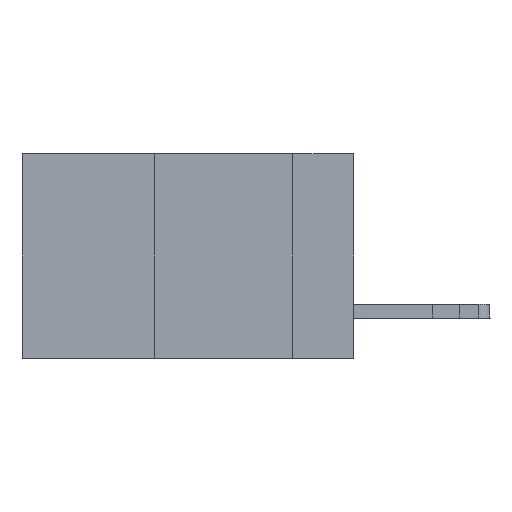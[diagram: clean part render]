
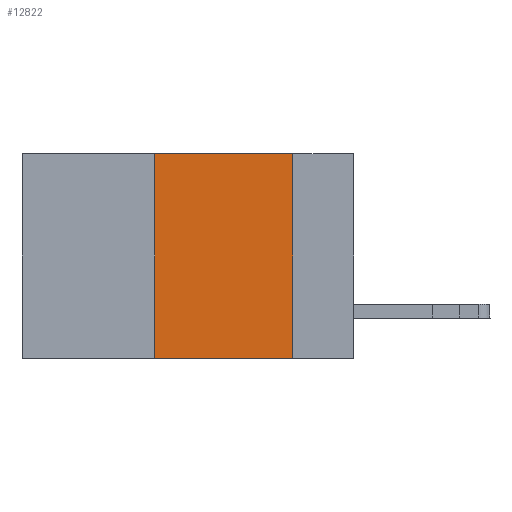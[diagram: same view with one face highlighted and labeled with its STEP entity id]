
A CAD part, left-side view. The second image highlights one B-rep face of the part: STEP entity #12822.
In plain terms, the highlighted planar face has unit normal (-1, 0, 0).
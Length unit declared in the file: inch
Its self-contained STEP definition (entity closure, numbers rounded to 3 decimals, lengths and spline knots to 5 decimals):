
#306 = ORIENTED_EDGE ( 'NONE', *, *, #20169, .F. ) ;
#942 = FACE_OUTER_BOUND ( 'NONE', #16333, .T. ) ;
#2393 = VERTEX_POINT ( 'NONE', #7620 ) ;
#2724 = PLANE ( 'NONE',  #6733 ) ;
#3853 = LINE ( 'NONE', #5769, #23176 ) ;
#4171 = ORIENTED_EDGE ( 'NONE', *, *, #15342, .F. ) ;
#5148 = VECTOR ( 'NONE', #10965, 39.37008 ) ;
#5769 = CARTESIAN_POINT ( 'NONE',  ( 0., 0.36, 0. ) ) ;
#5931 = VERTEX_POINT ( 'NONE', #22778 ) ;
#6733 = AXIS2_PLACEMENT_3D ( 'NONE', #22845, #21169, #19491 ) ;
#7384 = LINE ( 'NONE', #9068, #5148 ) ;
#7620 = CARTESIAN_POINT ( 'NONE',  ( 0., 0.36, 0. ) ) ;
#7730 = CARTESIAN_POINT ( 'NONE',  ( 0., 0.11, 0. ) ) ;
#7844 = VERTEX_POINT ( 'NONE', #20272 ) ;
#8581 = CARTESIAN_POINT ( 'NONE',  ( 0., 0.11, -0.37 ) ) ;
#8760 = ORIENTED_EDGE ( 'NONE', *, *, #23398, .F. ) ;
#9068 = CARTESIAN_POINT ( 'NONE',  ( 0., 0.6, -0.37 ) ) ;
#9505 = VECTOR ( 'NONE', #17516, 39.37008 ) ;
#10965 = DIRECTION ( 'NONE',  ( 0., -1., 0. ) ) ;
#11073 = VERTEX_POINT ( 'NONE', #8581 ) ;
#11653 = DIRECTION ( 'NONE',  ( 0., 0., -1. ) ) ;
#11854 = ORIENTED_EDGE ( 'NONE', *, *, #14132, .T. ) ;
#12822 = ADVANCED_FACE ( 'NONE', ( #942 ), #2724, .F. ) ;
#13293 = DIRECTION ( 'NONE',  ( 0., 0., 1. ) ) ;
#13681 = LINE ( 'NONE', #23028, #9505 ) ;
#14132 = EDGE_CURVE ( 'NONE', #7844, #11073, #7384, .T. ) ;
#15342 = EDGE_CURVE ( 'NONE', #7844, #2393, #3853, .T. ) ;
#15755 = VECTOR ( 'NONE', #11653, 39.37008 ) ;
#16333 = EDGE_LOOP ( 'NONE', ( #8760, #306, #4171, #11854 ) ) ;
#17516 = DIRECTION ( 'NONE',  ( 0., -1., 0. ) ) ;
#19491 = DIRECTION ( 'NONE',  ( 0., 0., -1. ) ) ;
#20169 = EDGE_CURVE ( 'NONE', #2393, #5931, #13681, .T. ) ;
#20272 = CARTESIAN_POINT ( 'NONE',  ( 0., 0.36, -0.37 ) ) ;
#20431 = LINE ( 'NONE', #7730, #15755 ) ;
#21169 = DIRECTION ( 'NONE',  ( 1., 0., 0. ) ) ;
#22778 = CARTESIAN_POINT ( 'NONE',  ( 0., 0.11, 0. ) ) ;
#22845 = CARTESIAN_POINT ( 'NONE',  ( 0., 0.6, 0. ) ) ;
#23028 = CARTESIAN_POINT ( 'NONE',  ( 0., 0.6, 0. ) ) ;
#23176 = VECTOR ( 'NONE', #13293, 39.37008 ) ;
#23398 = EDGE_CURVE ( 'NONE', #5931, #11073, #20431, .T. ) ;
